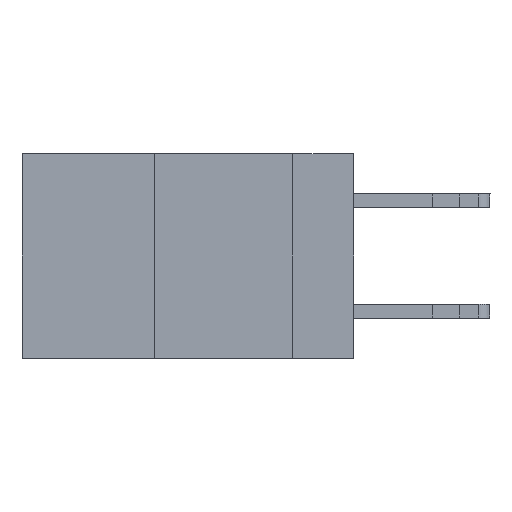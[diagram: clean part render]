
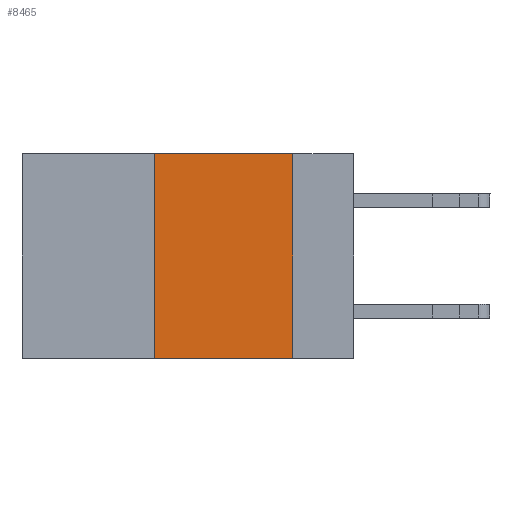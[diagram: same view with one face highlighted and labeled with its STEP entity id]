
A CAD part, left-side view. The second image highlights one B-rep face of the part: STEP entity #8465.
In plain terms, the highlighted planar face has unit normal (-1, 0, 0).
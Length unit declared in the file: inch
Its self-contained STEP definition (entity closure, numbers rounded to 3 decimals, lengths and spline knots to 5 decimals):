
#860 = ORIENTED_EDGE ( 'NONE', *, *, #16818, .F. ) ;
#1296 = ORIENTED_EDGE ( 'NONE', *, *, #6413, .F. ) ;
#1405 = CARTESIAN_POINT ( 'NONE',  ( 0., 0.6, 0. ) ) ;
#1712 = CARTESIAN_POINT ( 'NONE',  ( 0., 0.11, 0. ) ) ;
#1951 = EDGE_LOOP ( 'NONE', ( #860, #21596, #1296, #19506 ) ) ;
#2310 = VECTOR ( 'NONE', #10226, 39.37008 ) ;
#2452 = CARTESIAN_POINT ( 'NONE',  ( 0., 0.36, 0. ) ) ;
#3326 = LINE ( 'NONE', #1405, #2310 ) ;
#4083 = CARTESIAN_POINT ( 'NONE',  ( 0., 0.11, -0.37 ) ) ;
#4602 = AXIS2_PLACEMENT_3D ( 'NONE', #20981, #21093, #16855 ) ;
#5128 = CARTESIAN_POINT ( 'NONE',  ( 0., 0.6, -0.37 ) ) ;
#6089 = CARTESIAN_POINT ( 'NONE',  ( 0., 0.36, -0.37 ) ) ;
#6413 = EDGE_CURVE ( 'NONE', #22045, #10654, #12749, .T. ) ;
#7967 = VECTOR ( 'NONE', #10323, 39.37008 ) ;
#8273 = VERTEX_POINT ( 'NONE', #4083 ) ;
#8465 = ADVANCED_FACE ( 'NONE', ( #15889 ), #14064, .F. ) ;
#9555 = CARTESIAN_POINT ( 'NONE',  ( 0., 0.36, 0. ) ) ;
#9821 = LINE ( 'NONE', #13446, #17472 ) ;
#10226 = DIRECTION ( 'NONE',  ( 0., -1., 0. ) ) ;
#10323 = DIRECTION ( 'NONE',  ( 0., -1., 0. ) ) ;
#10654 = VERTEX_POINT ( 'NONE', #9555 ) ;
#12381 = EDGE_CURVE ( 'NONE', #22045, #8273, #20646, .T. ) ;
#12749 = LINE ( 'NONE', #2452, #14349 ) ;
#13446 = CARTESIAN_POINT ( 'NONE',  ( 0., 0.11, 0. ) ) ;
#14064 = PLANE ( 'NONE',  #4602 ) ;
#14349 = VECTOR ( 'NONE', #18309, 39.37008 ) ;
#15889 = FACE_OUTER_BOUND ( 'NONE', #1951, .T. ) ;
#16818 = EDGE_CURVE ( 'NONE', #19783, #8273, #9821, .T. ) ;
#16855 = DIRECTION ( 'NONE',  ( 0., 0., -1. ) ) ;
#17472 = VECTOR ( 'NONE', #22073, 39.37008 ) ;
#18309 = DIRECTION ( 'NONE',  ( 0., 0., 1. ) ) ;
#19506 = ORIENTED_EDGE ( 'NONE', *, *, #12381, .T. ) ;
#19783 = VERTEX_POINT ( 'NONE', #1712 ) ;
#20616 = EDGE_CURVE ( 'NONE', #10654, #19783, #3326, .T. ) ;
#20646 = LINE ( 'NONE', #5128, #7967 ) ;
#20981 = CARTESIAN_POINT ( 'NONE',  ( 0., 0.6, 0. ) ) ;
#21093 = DIRECTION ( 'NONE',  ( 1., 0., 0. ) ) ;
#21596 = ORIENTED_EDGE ( 'NONE', *, *, #20616, .F. ) ;
#22045 = VERTEX_POINT ( 'NONE', #6089 ) ;
#22073 = DIRECTION ( 'NONE',  ( 0., 0., -1. ) ) ;
